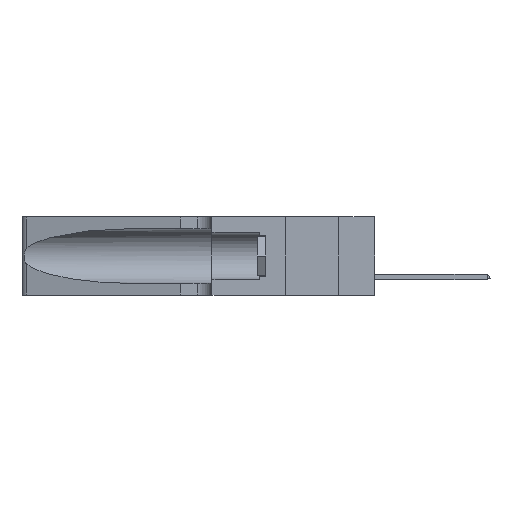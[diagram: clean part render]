
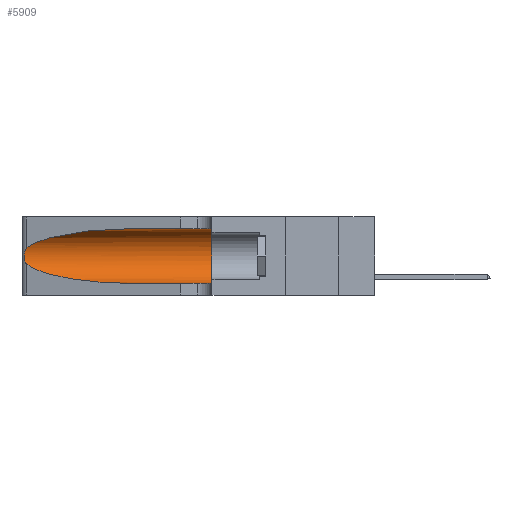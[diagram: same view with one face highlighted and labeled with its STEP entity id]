
A CAD part, left-side view. The second image highlights one B-rep face of the part: STEP entity #5909.
In plain terms, the highlighted cylindrical face has radius 3.308 mm (diameter 6.617 mm), a partial arc.
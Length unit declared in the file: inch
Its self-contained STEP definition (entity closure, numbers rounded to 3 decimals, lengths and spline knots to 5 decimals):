
#999 = EDGE_CURVE ( 'NONE', #25286, #28005, #11439, .T. ) ;
#1420 = ORIENTED_EDGE ( 'NONE', *, *, #10211, .F. ) ;
#2027 = DIRECTION ( 'NONE',  ( 0., 1., 0. ) ) ;
#2106 = CARTESIAN_POINT ( 'NONE',  ( 0.25487, 1.22718, 0.14631 ) ) ;
#2388 = CARTESIAN_POINT ( 'NONE',  ( 0.18966, 0.96281, 0.05475 ) ) ;
#2596 = CARTESIAN_POINT ( 'NONE',  ( 0.26075, 1.23896, 0.178 ) ) ;
#2887 = CARTESIAN_POINT ( 'NONE',  ( 0.1305, 0.72297, 0.05475 ) ) ;
#5047 = CARTESIAN_POINT ( 'NONE',  ( 0.25487, 1.22718, 0.14631 ) ) ;
#5122 = CARTESIAN_POINT ( 'NONE',  ( 0.1305, 0.72297, 0.31525 ) ) ;
#5328 = CARTESIAN_POINT ( 'NONE',  ( 0.2373, 1.15595, 0.28018 ) ) ;
#5355 = CARTESIAN_POINT ( 'NONE',  ( 0.26017, 1.23833, 0.17102 ) ) ;
#5612 = CARTESIAN_POINT ( 'NONE',  ( 0.1305, 1.61858, 0.185 ) ) ;
#5909 = ADVANCED_FACE ( 'NONE', ( #8288 ), #24680, .F. ) ;
#6293 = CARTESIAN_POINT ( 'NONE',  ( 0.1305, 0.72297, 0.05475 ) ) ;
#7923 = CIRCLE ( 'NONE', #7940, 0.13025 ) ;
#7940 = AXIS2_PLACEMENT_3D ( 'NONE', #25248, #2027, #11171 ) ;
#8288 = FACE_OUTER_BOUND ( 'NONE', #24015, .T. ) ;
#9391 = CARTESIAN_POINT ( 'NONE',  ( 0.25787, 1.23484, 0.2124 ) ) ;
#9511 = VECTOR ( 'NONE', #28352, 39.37008 ) ;
#9564 = CARTESIAN_POINT ( 'NONE',  ( 0.18966, 0.96281, 0.31525 ) ) ;
#9716 = CARTESIAN_POINT ( 'NONE',  ( 0.1305, 0.35, 0.05475 ) ) ;
#10211 = EDGE_CURVE ( 'NONE', #25286, #26550, #19062, .T. ) ;
#10317 = VECTOR ( 'NONE', #27843, 39.37008 ) ;
#11002 = LINE ( 'NONE', #12016, #9511 ) ;
#11113 = CARTESIAN_POINT ( 'NONE',  ( 0.1305, 1.61858, 0.31525 ) ) ;
#11171 = DIRECTION ( 'NONE',  ( 0., 0., 1. ) ) ;
#11439 =( BOUNDED_CURVE ( )  B_SPLINE_CURVE ( 3, ( #5122, #9564, #5328, #21611 ),
 .UNSPECIFIED., .F., .F. ) 
 B_SPLINE_CURVE_WITH_KNOTS ( ( 4, 4 ),
 ( 1.5708, 2.84003 ),
 .UNSPECIFIED. ) 
 CURVE ( )  GEOMETRIC_REPRESENTATION_ITEM ( )  RATIONAL_B_SPLINE_CURVE ( ( 1., 0.87, 0.87, 1. ) ) 
 REPRESENTATION_ITEM ( '' )  );
#11647 = CARTESIAN_POINT ( 'NONE',  ( 0.25487, 1.22718, 0.14631 ) ) ;
#11834 = CARTESIAN_POINT ( 'NONE',  ( 0.25854, 1.2359, 0.20912 ) ) ;
#12016 = CARTESIAN_POINT ( 'NONE',  ( 0.1305, 1.61858, 0.05475 ) ) ;
#13045 = VERTEX_POINT ( 'NONE', #11647 ) ;
#13738 = EDGE_CURVE ( 'NONE', #13045, #17774, #20938, .T. ) ;
#14181 = CARTESIAN_POINT ( 'NONE',  ( 0.26018, 1.23835, 0.19895 ) ) ;
#14439 = EDGE_CURVE ( 'NONE', #26550, #28479, #7923, .T. ) ;
#16523 = CARTESIAN_POINT ( 'NONE',  ( 0.26075, 1.23896, 0.19203 ) ) ;
#16728 = CARTESIAN_POINT ( 'NONE',  ( 0.25789, 1.23486, 0.15765 ) ) ;
#17774 = VERTEX_POINT ( 'NONE', #6293 ) ;
#18195 = EDGE_CURVE ( 'NONE', #17774, #28479, #11002, .T. ) ;
#18490 = ORIENTED_EDGE ( 'NONE', *, *, #21858, .T. ) ;
#18657 = CARTESIAN_POINT ( 'NONE',  ( 0.25555, 1.22994, 0.2215 ) ) ;
#18689 = B_SPLINE_CURVE_WITH_KNOTS ( 'NONE', 3,
 ( #25793, #18657, #21011, #9391, #11834, #14181, #16523, #2596, #5355, #26433, #16728, #19281, #19070, #5047 ),
 .UNSPECIFIED., .F., .F.,
 ( 4, 2, 2, 2, 2, 2, 4 ),
 ( 0., 0.00027, 0.00053, 0.00107, 0.0016, 0.00187, 0.00214 ),
 .UNSPECIFIED. ) ;
#19062 = LINE ( 'NONE', #11113, #10317 ) ;
#19070 = CARTESIAN_POINT ( 'NONE',  ( 0.25555, 1.22993, 0.14849 ) ) ;
#19281 = CARTESIAN_POINT ( 'NONE',  ( 0.25639, 1.23186, 0.15144 ) ) ;
#19325 = DIRECTION ( 'NONE',  ( 0., -1., 0. ) ) ;
#20421 = ORIENTED_EDGE ( 'NONE', *, *, #18195, .T. ) ;
#20788 = ORIENTED_EDGE ( 'NONE', *, *, #13738, .T. ) ;
#20863 = CARTESIAN_POINT ( 'NONE',  ( 0.1305, 0.72297, 0.31525 ) ) ;
#20938 =( BOUNDED_CURVE ( )  B_SPLINE_CURVE ( 3, ( #2106, #23258, #2388, #2887 ),
 .UNSPECIFIED., .F., .F. ) 
 B_SPLINE_CURVE_WITH_KNOTS ( ( 4, 4 ),
 ( 3.44316, 4.71239 ),
 .UNSPECIFIED. ) 
 CURVE ( )  GEOMETRIC_REPRESENTATION_ITEM ( )  RATIONAL_B_SPLINE_CURVE ( ( 1., 0.87, 0.87, 1. ) ) 
 REPRESENTATION_ITEM ( '' )  );
#21011 = CARTESIAN_POINT ( 'NONE',  ( 0.25639, 1.23184, 0.21858 ) ) ;
#21611 = CARTESIAN_POINT ( 'NONE',  ( 0.25487, 1.22718, 0.22369 ) ) ;
#21858 = EDGE_CURVE ( 'NONE', #28005, #13045, #18689, .T. ) ;
#23258 = CARTESIAN_POINT ( 'NONE',  ( 0.2373, 1.15595, 0.08982 ) ) ;
#23367 = ORIENTED_EDGE ( 'NONE', *, *, #999, .T. ) ;
#24015 = EDGE_LOOP ( 'NONE', ( #23367, #18490, #20788, #20421, #24602, #1420 ) ) ;
#24563 = CARTESIAN_POINT ( 'NONE',  ( 0.1305, 0.35, 0.31525 ) ) ;
#24602 = ORIENTED_EDGE ( 'NONE', *, *, #14439, .F. ) ;
#24680 = CYLINDRICAL_SURFACE ( 'NONE', #28867, 0.13025 ) ;
#25248 = CARTESIAN_POINT ( 'NONE',  ( 0.1305, 0.35, 0.185 ) ) ;
#25286 = VERTEX_POINT ( 'NONE', #20863 ) ;
#25793 = CARTESIAN_POINT ( 'NONE',  ( 0.25487, 1.22718, 0.22369 ) ) ;
#26370 = DIRECTION ( 'NONE',  ( 0., 0., -1. ) ) ;
#26433 = CARTESIAN_POINT ( 'NONE',  ( 0.25856, 1.23593, 0.16098 ) ) ;
#26550 = VERTEX_POINT ( 'NONE', #24563 ) ;
#27843 = DIRECTION ( 'NONE',  ( 0., -1., 0. ) ) ;
#28005 = VERTEX_POINT ( 'NONE', #29622 ) ;
#28352 = DIRECTION ( 'NONE',  ( 0., -1., 0. ) ) ;
#28479 = VERTEX_POINT ( 'NONE', #9716 ) ;
#28867 = AXIS2_PLACEMENT_3D ( 'NONE', #5612, #19325, #26370 ) ;
#29622 = CARTESIAN_POINT ( 'NONE',  ( 0.25487, 1.22718, 0.22369 ) ) ;
